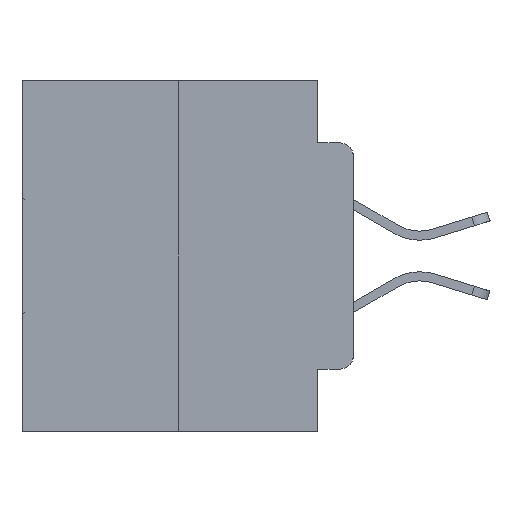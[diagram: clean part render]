
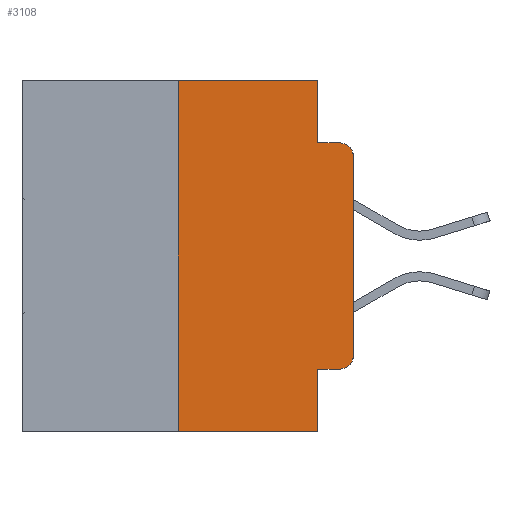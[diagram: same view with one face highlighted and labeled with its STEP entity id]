
A CAD part, left-side view. The second image highlights one B-rep face of the part: STEP entity #3108.
In plain terms, the highlighted planar face has unit normal (-1, 0, 0).
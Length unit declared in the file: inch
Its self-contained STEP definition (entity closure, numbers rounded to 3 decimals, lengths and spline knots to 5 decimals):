
#61 = LINE ( 'NONE', #7226, #18320 ) ;
#500 = CARTESIAN_POINT ( 'NONE',  ( 0., 0.02, -0.3915 ) ) ;
#506 = CARTESIAN_POINT ( 'NONE',  ( 0., 0.051, -0.4115 ) ) ;
#602 = LINE ( 'NONE', #28094, #17327 ) ;
#901 = CARTESIAN_POINT ( 'NONE',  ( 0., 0.25, 0. ) ) ;
#1153 = CARTESIAN_POINT ( 'NONE',  ( 0., 0., -0.1085 ) ) ;
#1561 = AXIS2_PLACEMENT_3D ( 'NONE', #500, #17144, #3000 ) ;
#1683 = DIRECTION ( 'NONE',  ( 0., -1., 0. ) ) ;
#1900 = DIRECTION ( 'NONE',  ( 0., 0., -1. ) ) ;
#2054 = CARTESIAN_POINT ( 'NONE',  ( 0., 0., -0.3915 ) ) ;
#3000 = DIRECTION ( 'NONE',  ( 0., 0., -1. ) ) ;
#3108 = ADVANCED_FACE ( 'NONE', ( #5877 ), #11404, .F. ) ;
#3132 = VECTOR ( 'NONE', #24417, 39.37008 ) ;
#3372 = DIRECTION ( 'NONE',  ( 0., 0., 1. ) ) ;
#3984 = EDGE_CURVE ( 'NONE', #24210, #8298, #61, .T. ) ;
#4067 = VERTEX_POINT ( 'NONE', #12253 ) ;
#4673 = VECTOR ( 'NONE', #12442, 39.37008 ) ;
#5871 = ORIENTED_EDGE ( 'NONE', *, *, #3984, .T. ) ;
#5877 = FACE_OUTER_BOUND ( 'NONE', #30360, .T. ) ;
#5960 = ORIENTED_EDGE ( 'NONE', *, *, #12563, .T. ) ;
#6170 = ORIENTED_EDGE ( 'NONE', *, *, #23466, .F. ) ;
#6287 = VECTOR ( 'NONE', #3372, 39.37008 ) ;
#6392 = ORIENTED_EDGE ( 'NONE', *, *, #29094, .F. ) ;
#6485 = ORIENTED_EDGE ( 'NONE', *, *, #6667, .F. ) ;
#6517 = ORIENTED_EDGE ( 'NONE', *, *, #27535, .F. ) ;
#6667 = EDGE_CURVE ( 'NONE', #25876, #4067, #602, .T. ) ;
#6870 = ORIENTED_EDGE ( 'NONE', *, *, #29595, .T. ) ;
#6990 = ORIENTED_EDGE ( 'NONE', *, *, #28295, .F. ) ;
#7217 = ORIENTED_EDGE ( 'NONE', *, *, #15957, .T. ) ;
#7226 = CARTESIAN_POINT ( 'NONE',  ( 0., 0., 0. ) ) ;
#7272 = ORIENTED_EDGE ( 'NONE', *, *, #14084, .T. ) ;
#7976 = CARTESIAN_POINT ( 'NONE',  ( 0., 0.473, -0.5 ) ) ;
#8298 = VERTEX_POINT ( 'NONE', #1153 ) ;
#8555 = CARTESIAN_POINT ( 'NONE',  ( 0., 0.051, 0. ) ) ;
#9233 = VERTEX_POINT ( 'NONE', #15612 ) ;
#10373 = DIRECTION ( 'NONE',  ( 0., -1., 0. ) ) ;
#10578 = VERTEX_POINT ( 'NONE', #20535 ) ;
#10980 = LINE ( 'NONE', #506, #4673 ) ;
#11200 = CARTESIAN_POINT ( 'NONE',  ( 0., 0.02, -0.1085 ) ) ;
#11404 = PLANE ( 'NONE',  #14532 ) ;
#11980 = CARTESIAN_POINT ( 'NONE',  ( 0., 0.051, -0.5 ) ) ;
#12253 = CARTESIAN_POINT ( 'NONE',  ( 0., 0.051, 0. ) ) ;
#12442 = DIRECTION ( 'NONE',  ( 0., -1., 0. ) ) ;
#12563 = EDGE_CURVE ( 'NONE', #8298, #19677, #16337, .T. ) ;
#12738 = CARTESIAN_POINT ( 'NONE',  ( 0., 0.051, 0. ) ) ;
#13594 = DIRECTION ( 'NONE',  ( 0., 0., -1. ) ) ;
#13602 = LINE ( 'NONE', #20516, #25289 ) ;
#13801 = CARTESIAN_POINT ( 'NONE',  ( 0., 0.473, 0. ) ) ;
#14084 = EDGE_CURVE ( 'NONE', #25509, #24210, #25034, .T. ) ;
#14532 = AXIS2_PLACEMENT_3D ( 'NONE', #13801, #25432, #1900 ) ;
#15612 = CARTESIAN_POINT ( 'NONE',  ( 0., 0.051, -0.4115 ) ) ;
#15734 = LINE ( 'NONE', #12738, #3132 ) ;
#15957 = EDGE_CURVE ( 'NONE', #9233, #25509, #10980, .T. ) ;
#16337 = CIRCLE ( 'NONE', #24098, 0.02 ) ;
#16591 = VECTOR ( 'NONE', #22586, 39.37008 ) ;
#17144 = DIRECTION ( 'NONE',  ( -1., 0., 0. ) ) ;
#17320 = VERTEX_POINT ( 'NONE', #28871 ) ;
#17327 = VECTOR ( 'NONE', #21137, 39.37008 ) ;
#18320 = VECTOR ( 'NONE', #25980, 39.37008 ) ;
#19357 = VECTOR ( 'NONE', #10373, 39.37008 ) ;
#19677 = VERTEX_POINT ( 'NONE', #21496 ) ;
#20516 = CARTESIAN_POINT ( 'NONE',  ( 0., 0.051, -0.0885 ) ) ;
#20535 = CARTESIAN_POINT ( 'NONE',  ( 0., 0.051, -0.0885 ) ) ;
#21117 = CARTESIAN_POINT ( 'NONE',  ( 0., 0.02, -0.4115 ) ) ;
#21137 = DIRECTION ( 'NONE',  ( 0., -1., 0. ) ) ;
#21496 = CARTESIAN_POINT ( 'NONE',  ( 0., 0.02, -0.0885 ) ) ;
#22586 = DIRECTION ( 'NONE',  ( 0., 0., -1. ) ) ;
#23466 = EDGE_CURVE ( 'NONE', #10578, #19677, #13602, .T. ) ;
#24098 = AXIS2_PLACEMENT_3D ( 'NONE', #11200, #27559, #13594 ) ;
#24210 = VERTEX_POINT ( 'NONE', #2054 ) ;
#24417 = DIRECTION ( 'NONE',  ( 0., 0., -1. ) ) ;
#25033 = LINE ( 'NONE', #901, #6287 ) ;
#25034 = CIRCLE ( 'NONE', #1561, 0.02 ) ;
#25289 = VECTOR ( 'NONE', #1683, 39.37008 ) ;
#25432 = DIRECTION ( 'NONE',  ( 1., 0., 0. ) ) ;
#25509 = VERTEX_POINT ( 'NONE', #21117 ) ;
#25876 = VERTEX_POINT ( 'NONE', #29635 ) ;
#25920 = LINE ( 'NONE', #7976, #19357 ) ;
#25980 = DIRECTION ( 'NONE',  ( 0., 0., 1. ) ) ;
#27535 = EDGE_CURVE ( 'NONE', #17320, #25876, #25033, .T. ) ;
#27559 = DIRECTION ( 'NONE',  ( -1., 0., 0. ) ) ;
#28094 = CARTESIAN_POINT ( 'NONE',  ( 0., 0.473, 0. ) ) ;
#28295 = EDGE_CURVE ( 'NONE', #9233, #29418, #28299, .T. ) ;
#28299 = LINE ( 'NONE', #8555, #16591 ) ;
#28871 = CARTESIAN_POINT ( 'NONE',  ( 0., 0.25, -0.5 ) ) ;
#29094 = EDGE_CURVE ( 'NONE', #4067, #10578, #15734, .T. ) ;
#29418 = VERTEX_POINT ( 'NONE', #11980 ) ;
#29595 = EDGE_CURVE ( 'NONE', #17320, #29418, #25920, .T. ) ;
#29635 = CARTESIAN_POINT ( 'NONE',  ( 0., 0.25, 0. ) ) ;
#30360 = EDGE_LOOP ( 'NONE', ( #5871, #5960, #6170, #6392, #6485, #6517, #6870, #6990, #7217, #7272 ) ) ;
